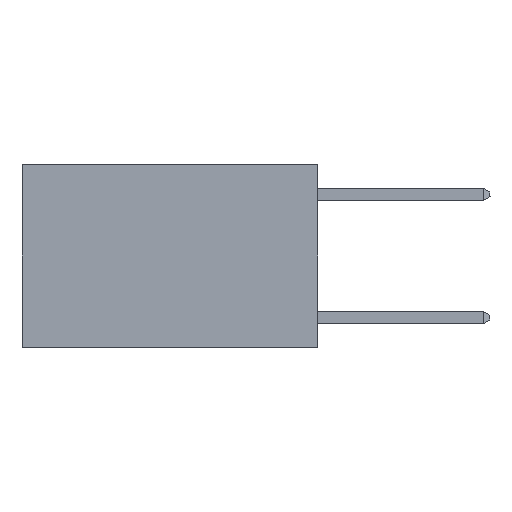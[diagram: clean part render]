
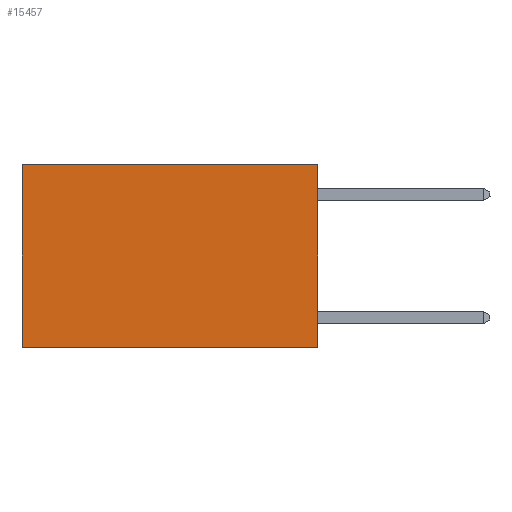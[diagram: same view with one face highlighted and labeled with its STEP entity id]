
A CAD part, left-side view. The second image highlights one B-rep face of the part: STEP entity #15457.
In plain terms, the highlighted planar face has unit normal (-1, 0, 0).
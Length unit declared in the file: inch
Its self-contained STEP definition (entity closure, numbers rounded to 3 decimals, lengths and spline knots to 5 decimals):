
#244 = EDGE_CURVE ( 'NONE', #16386, #15221, #4486, .T. ) ;
#2114 = DIRECTION ( 'NONE',  ( 0., 0., -1. ) ) ;
#2291 = EDGE_LOOP ( 'NONE', ( #10685, #24273, #3512, #21697 ) ) ;
#2295 = VECTOR ( 'NONE', #16852, 39.37008 ) ;
#2334 = VECTOR ( 'NONE', #4172, 39.37008 ) ;
#3512 = ORIENTED_EDGE ( 'NONE', *, *, #10705, .F. ) ;
#3884 = CARTESIAN_POINT ( 'NONE',  ( 0.2625, 0.6, 0. ) ) ;
#4172 = DIRECTION ( 'NONE',  ( 0., 1., 0. ) ) ;
#4200 = AXIS2_PLACEMENT_3D ( 'NONE', #12949, #7212, #12789 ) ;
#4486 = LINE ( 'NONE', #16776, #14890 ) ;
#4743 = LINE ( 'NONE', #21117, #2334 ) ;
#5358 = CARTESIAN_POINT ( 'NONE',  ( 0.2625, 0.6, -0.37 ) ) ;
#5458 = LINE ( 'NONE', #13539, #21767 ) ;
#6808 = EDGE_CURVE ( 'NONE', #22038, #21272, #4743, .T. ) ;
#7212 = DIRECTION ( 'NONE',  ( 1., 0., 0. ) ) ;
#10685 = ORIENTED_EDGE ( 'NONE', *, *, #21171, .T. ) ;
#10705 = EDGE_CURVE ( 'NONE', #16386, #22038, #5458, .T. ) ;
#12789 = DIRECTION ( 'NONE',  ( 0., 0., -1. ) ) ;
#12949 = CARTESIAN_POINT ( 'NONE',  ( 0.2625, 0., 0. ) ) ;
#13539 = CARTESIAN_POINT ( 'NONE',  ( 0.2625, 0., 0. ) ) ;
#14890 = VECTOR ( 'NONE', #16859, 39.37008 ) ;
#15221 = VERTEX_POINT ( 'NONE', #23373 ) ;
#15457 = ADVANCED_FACE ( 'NONE', ( #21648 ), #22484, .F. ) ;
#16386 = VERTEX_POINT ( 'NONE', #19609 ) ;
#16776 = CARTESIAN_POINT ( 'NONE',  ( 0.2625, 0., 0. ) ) ;
#16852 = DIRECTION ( 'NONE',  ( 0., 0., -1. ) ) ;
#16859 = DIRECTION ( 'NONE',  ( 0., 1., 0. ) ) ;
#19609 = CARTESIAN_POINT ( 'NONE',  ( 0.2625, 0., 0. ) ) ;
#20327 = CARTESIAN_POINT ( 'NONE',  ( 0.2625, 0., -0.37 ) ) ;
#21117 = CARTESIAN_POINT ( 'NONE',  ( 0.2625, 0., -0.37 ) ) ;
#21171 = EDGE_CURVE ( 'NONE', #15221, #21272, #22526, .T. ) ;
#21272 = VERTEX_POINT ( 'NONE', #5358 ) ;
#21648 = FACE_OUTER_BOUND ( 'NONE', #2291, .T. ) ;
#21697 = ORIENTED_EDGE ( 'NONE', *, *, #244, .T. ) ;
#21767 = VECTOR ( 'NONE', #2114, 39.37008 ) ;
#22038 = VERTEX_POINT ( 'NONE', #20327 ) ;
#22484 = PLANE ( 'NONE',  #4200 ) ;
#22526 = LINE ( 'NONE', #3884, #2295 ) ;
#23373 = CARTESIAN_POINT ( 'NONE',  ( 0.2625, 0.6, 0. ) ) ;
#24273 = ORIENTED_EDGE ( 'NONE', *, *, #6808, .F. ) ;
